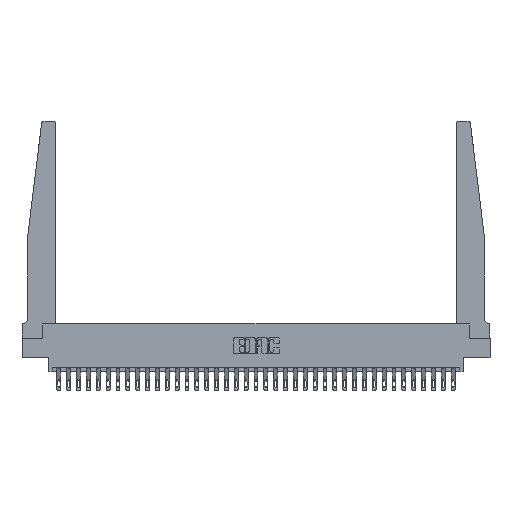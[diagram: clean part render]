
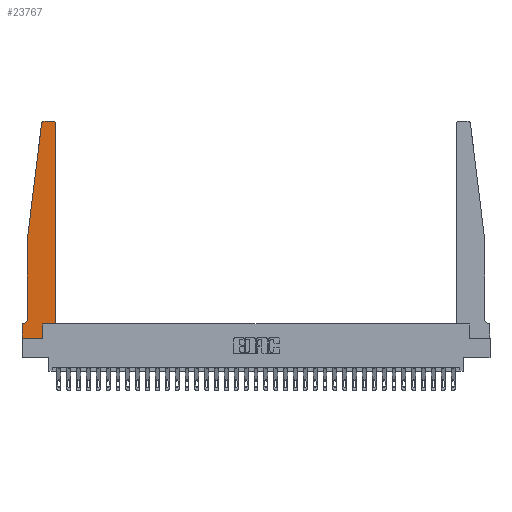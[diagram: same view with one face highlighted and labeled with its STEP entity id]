
A CAD part, top view. The second image highlights one B-rep face of the part: STEP entity #23767.
In plain terms, the highlighted planar face has unit normal (0, 0, 1).
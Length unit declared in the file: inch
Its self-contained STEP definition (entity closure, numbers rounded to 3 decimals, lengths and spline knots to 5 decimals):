
#330 = ORIENTED_EDGE ( 'NONE', *, *, #22133, .T. ) ;
#334 = DIRECTION ( 'NONE',  ( 0., -1., 0. ) ) ;
#511 = DIRECTION ( 'NONE',  ( 0., 0., 1. ) ) ;
#841 = DIRECTION ( 'NONE',  ( 1., 0., 0. ) ) ;
#943 = EDGE_CURVE ( 'NONE', #9704, #28652, #1336, .T. ) ;
#1336 = CIRCLE ( 'NONE', #23421, 0.03 ) ;
#1638 = DIRECTION ( 'NONE',  ( -0.122, -0.992, 0. ) ) ;
#2611 = VERTEX_POINT ( 'NONE', #14579 ) ;
#2808 = ORIENTED_EDGE ( 'NONE', *, *, #20469, .T. ) ;
#2828 = CARTESIAN_POINT ( 'NONE',  ( 0.065, 0.2375, 0.37 ) ) ;
#2915 = DIRECTION ( 'NONE',  ( 1., 0., 0. ) ) ;
#4005 = ORIENTED_EDGE ( 'NONE', *, *, #22445, .T. ) ;
#4747 = CARTESIAN_POINT ( 'NONE',  ( 0.065, 1.25, 0.37 ) ) ;
#5187 = VERTEX_POINT ( 'NONE', #6365 ) ;
#5974 = CARTESIAN_POINT ( 'NONE',  ( 0.425, 0.18, 0.37 ) ) ;
#6365 = CARTESIAN_POINT ( 'NONE',  ( 0.2605, 0., 0.37 ) ) ;
#7085 = EDGE_CURVE ( 'NONE', #12986, #14733, #21326, .T. ) ;
#7121 = CARTESIAN_POINT ( 'NONE',  ( 0., 0., 0.37 ) ) ;
#7332 = CARTESIAN_POINT ( 'NONE',  ( 0.27653, 2.75, 0.37 ) ) ;
#7355 = CARTESIAN_POINT ( 'NONE',  ( 0.27653, 2.72, 0.37 ) ) ;
#7649 = ORIENTED_EDGE ( 'NONE', *, *, #20709, .T. ) ;
#7718 = DIRECTION ( 'NONE',  ( 1., 0., 0. ) ) ;
#7788 = VERTEX_POINT ( 'NONE', #31675 ) ;
#8307 = CARTESIAN_POINT ( 'NONE',  ( 0.425, 0.18, 0.37 ) ) ;
#8816 = ORIENTED_EDGE ( 'NONE', *, *, #15756, .T. ) ;
#9704 = VERTEX_POINT ( 'NONE', #7332 ) ;
#9760 = ORIENTED_EDGE ( 'NONE', *, *, #23913, .T. ) ;
#11247 = LINE ( 'NONE', #31357, #15382 ) ;
#11544 = VECTOR ( 'NONE', #13602, 39.37008 ) ;
#12894 = LINE ( 'NONE', #22914, #17002 ) ;
#12986 = VERTEX_POINT ( 'NONE', #5974 ) ;
#13602 = DIRECTION ( 'NONE',  ( 0., 1., 0. ) ) ;
#13883 = VECTOR ( 'NONE', #21387, 39.37008 ) ;
#14192 = LINE ( 'NONE', #24221, #16868 ) ;
#14440 = EDGE_CURVE ( 'NONE', #28652, #23814, #14192, .T. ) ;
#14579 = CARTESIAN_POINT ( 'NONE',  ( 0., 0.1875, 0.37 ) ) ;
#14733 = VERTEX_POINT ( 'NONE', #28156 ) ;
#15382 = VECTOR ( 'NONE', #18826, 39.37008 ) ;
#15453 = VERTEX_POINT ( 'NONE', #2828 ) ;
#15756 = EDGE_CURVE ( 'NONE', #28807, #2611, #32305, .T. ) ;
#16174 = CARTESIAN_POINT ( 'NONE',  ( 0.015, 0.1875, 0.37 ) ) ;
#16381 = ORIENTED_EDGE ( 'NONE', *, *, #30684, .T. ) ;
#16868 = VECTOR ( 'NONE', #1638, 39.37008 ) ;
#16978 = CIRCLE ( 'NONE', #26967, 0.05 ) ;
#17002 = VECTOR ( 'NONE', #334, 39.37008 ) ;
#17364 = DIRECTION ( 'NONE',  ( 0., -1., 0. ) ) ;
#17461 = LINE ( 'NONE', #20410, #22350 ) ;
#17843 = CARTESIAN_POINT ( 'NONE',  ( 0.395, 2.75, 0.37 ) ) ;
#17953 = CARTESIAN_POINT ( 'NONE',  ( 0., 0., 0.37 ) ) ;
#18081 = EDGE_LOOP ( 'NONE', ( #330, #20310, #22959, #26232, #4005, #8816, #2808, #16381, #9760, #32371, #26744, #7649 ) ) ;
#18297 = CARTESIAN_POINT ( 'NONE',  ( 0.015, 0.2375, 0.37 ) ) ;
#18577 = LINE ( 'NONE', #19337, #24080 ) ;
#18826 = DIRECTION ( 'NONE',  ( -1., 0., 0. ) ) ;
#19213 = VECTOR ( 'NONE', #17364, 39.37008 ) ;
#19337 = CARTESIAN_POINT ( 'NONE',  ( 0., 0., 0.37 ) ) ;
#19917 = FACE_OUTER_BOUND ( 'NONE', #18081, .T. ) ;
#20086 = DIRECTION ( 'NONE',  ( 0., 0., 1. ) ) ;
#20310 = ORIENTED_EDGE ( 'NONE', *, *, #943, .T. ) ;
#20410 = CARTESIAN_POINT ( 'NONE',  ( 0.425, 0.18, 0.37 ) ) ;
#20469 = EDGE_CURVE ( 'NONE', #2611, #27144, #24766, .T. ) ;
#20591 = DIRECTION ( 'NONE',  ( 0., 0., -1. ) ) ;
#20709 = EDGE_CURVE ( 'NONE', #14733, #29683, #29677, .T. ) ;
#20723 = AXIS2_PLACEMENT_3D ( 'NONE', #25905, #511, #841 ) ;
#21326 = LINE ( 'NONE', #8307, #11544 ) ;
#21387 = DIRECTION ( 'NONE',  ( 0., 1., 0. ) ) ;
#21772 = AXIS2_PLACEMENT_3D ( 'NONE', #23037, #20086, #7718 ) ;
#22133 = EDGE_CURVE ( 'NONE', #29683, #9704, #11247, .T. ) ;
#22350 = VECTOR ( 'NONE', #30474, 39.37008 ) ;
#22445 = EDGE_CURVE ( 'NONE', #15453, #28807, #16978, .T. ) ;
#22714 = VECTOR ( 'NONE', #29339, 39.37008 ) ;
#22766 = CARTESIAN_POINT ( 'NONE',  ( 0.24675, 2.72367, 0.37 ) ) ;
#22914 = CARTESIAN_POINT ( 'NONE',  ( 0.065, 1.25, 0.37 ) ) ;
#22959 = ORIENTED_EDGE ( 'NONE', *, *, #14440, .T. ) ;
#23037 = CARTESIAN_POINT ( 'NONE',  ( 0., 0.1875, 0.37 ) ) ;
#23063 = DIRECTION ( 'NONE',  ( -1., 0., 0. ) ) ;
#23372 = EDGE_CURVE ( 'NONE', #23814, #15453, #12894, .T. ) ;
#23421 = AXIS2_PLACEMENT_3D ( 'NONE', #7355, #27966, #2915 ) ;
#23691 = LINE ( 'NONE', #31293, #13883 ) ;
#23767 = ADVANCED_FACE ( 'NONE', ( #19917 ), #29968, .T. ) ;
#23814 = VERTEX_POINT ( 'NONE', #4747 ) ;
#23913 = EDGE_CURVE ( 'NONE', #5187, #7788, #23691, .T. ) ;
#24080 = VECTOR ( 'NONE', #29226, 39.37008 ) ;
#24221 = CARTESIAN_POINT ( 'NONE',  ( 0.065, 1.25, 0.37 ) ) ;
#24228 = CARTESIAN_POINT ( 'NONE',  ( 0.065, 0.1875, 0.37 ) ) ;
#24766 = LINE ( 'NONE', #7121, #19213 ) ;
#25905 = CARTESIAN_POINT ( 'NONE',  ( 0.395, 2.72, 0.37 ) ) ;
#26232 = ORIENTED_EDGE ( 'NONE', *, *, #23372, .T. ) ;
#26744 = ORIENTED_EDGE ( 'NONE', *, *, #7085, .T. ) ;
#26967 = AXIS2_PLACEMENT_3D ( 'NONE', #18297, #20591, #23063 ) ;
#27142 = EDGE_CURVE ( 'NONE', #7788, #12986, #17461, .T. ) ;
#27144 = VERTEX_POINT ( 'NONE', #17953 ) ;
#27966 = DIRECTION ( 'NONE',  ( 0., 0., 1. ) ) ;
#28156 = CARTESIAN_POINT ( 'NONE',  ( 0.425, 2.72, 0.37 ) ) ;
#28652 = VERTEX_POINT ( 'NONE', #22766 ) ;
#28807 = VERTEX_POINT ( 'NONE', #16174 ) ;
#29226 = DIRECTION ( 'NONE',  ( 1., 0., 0. ) ) ;
#29339 = DIRECTION ( 'NONE',  ( -1., 0., 0. ) ) ;
#29677 = CIRCLE ( 'NONE', #20723, 0.03 ) ;
#29683 = VERTEX_POINT ( 'NONE', #17843 ) ;
#29968 = PLANE ( 'NONE',  #21772 ) ;
#30474 = DIRECTION ( 'NONE',  ( 1., 0., 0. ) ) ;
#30684 = EDGE_CURVE ( 'NONE', #27144, #5187, #18577, .T. ) ;
#31293 = CARTESIAN_POINT ( 'NONE',  ( 0.2605, 0.18, 0.37 ) ) ;
#31357 = CARTESIAN_POINT ( 'NONE',  ( 0.25, 2.75, 0.37 ) ) ;
#31675 = CARTESIAN_POINT ( 'NONE',  ( 0.2605, 0.18, 0.37 ) ) ;
#32305 = LINE ( 'NONE', #24228, #22714 ) ;
#32371 = ORIENTED_EDGE ( 'NONE', *, *, #27142, .T. ) ;
